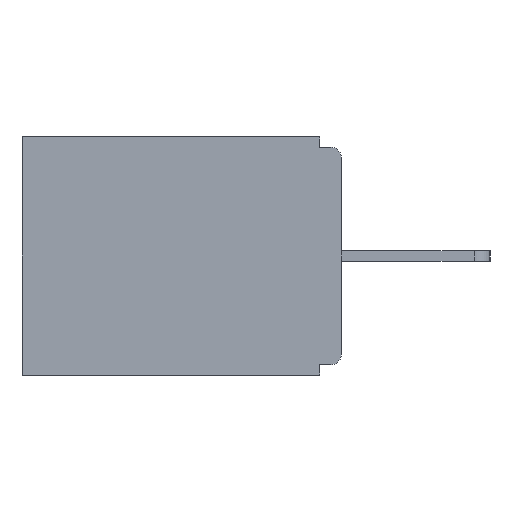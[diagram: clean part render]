
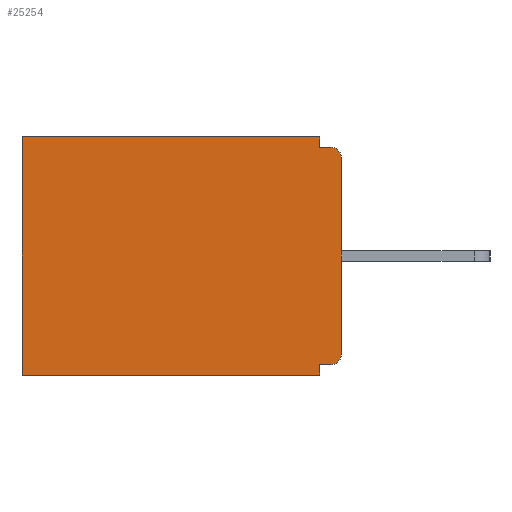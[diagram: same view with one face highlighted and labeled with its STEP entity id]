
A CAD part, left-side view. The second image highlights one B-rep face of the part: STEP entity #25254.
In plain terms, the highlighted planar face has unit normal (-1, 0, 0).
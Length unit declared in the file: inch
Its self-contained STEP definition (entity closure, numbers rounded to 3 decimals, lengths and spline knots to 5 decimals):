
#625 = DIRECTION ( 'NONE',  ( 0., 1., 0. ) ) ;
#708 = EDGE_CURVE ( 'NONE', #4098, #7398, #16030, .T. ) ;
#972 = PLANE ( 'NONE',  #22437 ) ;
#1460 = CARTESIAN_POINT ( 'NONE',  ( 0.298, 0., -0.343 ) ) ;
#1604 = VECTOR ( 'NONE', #17509, 39.37008 ) ;
#1806 = VECTOR ( 'NONE', #6865, 39.37008 ) ;
#1820 = DIRECTION ( 'NONE',  ( 0., 1., 0. ) ) ;
#1866 = ORIENTED_EDGE ( 'NONE', *, *, #15535, .F. ) ;
#1882 = EDGE_CURVE ( 'NONE', #14645, #4284, #15303, .T. ) ;
#1929 = CARTESIAN_POINT ( 'NONE',  ( 0.298, 0.015, -0.313 ) ) ;
#2220 = CARTESIAN_POINT ( 'NONE',  ( 0.298, 0.031, -0.015 ) ) ;
#2470 = EDGE_CURVE ( 'NONE', #3941, #7398, #4201, .T. ) ;
#2861 = DIRECTION ( 'NONE',  ( 0., 0., -1. ) ) ;
#2925 = DIRECTION ( 'NONE',  ( 0., 0., -1. ) ) ;
#3166 = FACE_OUTER_BOUND ( 'NONE', #17332, .T. ) ;
#3941 = VERTEX_POINT ( 'NONE', #17111 ) ;
#4076 = DIRECTION ( 'NONE',  ( 0., 0., -1. ) ) ;
#4098 = VERTEX_POINT ( 'NONE', #25697 ) ;
#4145 = ORIENTED_EDGE ( 'NONE', *, *, #6906, .T. ) ;
#4201 = LINE ( 'NONE', #1460, #8117 ) ;
#4284 = VERTEX_POINT ( 'NONE', #16744 ) ;
#4584 = VECTOR ( 'NONE', #2861, 39.37008 ) ;
#4990 = CARTESIAN_POINT ( 'NONE',  ( 0.298, 0.031, -0.328 ) ) ;
#4994 = ORIENTED_EDGE ( 'NONE', *, *, #20218, .F. ) ;
#5400 = CARTESIAN_POINT ( 'NONE',  ( 0.298, 0.46, -0.343 ) ) ;
#5636 = AXIS2_PLACEMENT_3D ( 'NONE', #26650, #8255, #4076 ) ;
#5731 = ORIENTED_EDGE ( 'NONE', *, *, #1882, .T. ) ;
#6865 = DIRECTION ( 'NONE',  ( 0., 0., -1. ) ) ;
#6906 = EDGE_CURVE ( 'NONE', #20373, #4098, #23483, .T. ) ;
#7398 = VERTEX_POINT ( 'NONE', #5400 ) ;
#8070 = ORIENTED_EDGE ( 'NONE', *, *, #24439, .F. ) ;
#8078 = ORIENTED_EDGE ( 'NONE', *, *, #12468, .F. ) ;
#8117 = VECTOR ( 'NONE', #1820, 39.37008 ) ;
#8255 = DIRECTION ( 'NONE',  ( -1., 0., 0. ) ) ;
#9333 = CARTESIAN_POINT ( 'NONE',  ( 0.298, 0., 0. ) ) ;
#10037 = CARTESIAN_POINT ( 'NONE',  ( 0.298, 0., -0.03 ) ) ;
#10203 = ORIENTED_EDGE ( 'NONE', *, *, #2470, .F. ) ;
#11081 = CARTESIAN_POINT ( 'NONE',  ( 0.298, 0.015, -0.015 ) ) ;
#11127 = VECTOR ( 'NONE', #625, 39.37008 ) ;
#11611 = DIRECTION ( 'NONE',  ( 0., -1., 0. ) ) ;
#11946 = VERTEX_POINT ( 'NONE', #10037 ) ;
#12468 = EDGE_CURVE ( 'NONE', #21699, #15199, #17417, .T. ) ;
#13054 = ORIENTED_EDGE ( 'NONE', *, *, #23594, .T. ) ;
#13057 = CARTESIAN_POINT ( 'NONE',  ( 0.298, 0., -0.328 ) ) ;
#13523 = CARTESIAN_POINT ( 'NONE',  ( 0.298, 0.031, -0.343 ) ) ;
#14033 = LINE ( 'NONE', #15560, #4584 ) ;
#14142 = CARTESIAN_POINT ( 'NONE',  ( 0.298, 0.015, -0.328 ) ) ;
#14493 = VECTOR ( 'NONE', #15778, 39.37008 ) ;
#14543 = CIRCLE ( 'NONE', #5636, 0.015 ) ;
#14645 = VERTEX_POINT ( 'NONE', #14142 ) ;
#15199 = VERTEX_POINT ( 'NONE', #11081 ) ;
#15303 = CIRCLE ( 'NONE', #17388, 0.015 ) ;
#15433 = CARTESIAN_POINT ( 'NONE',  ( 0.298, 0., 0. ) ) ;
#15535 = EDGE_CURVE ( 'NONE', #11946, #4284, #20571, .T. ) ;
#15560 = CARTESIAN_POINT ( 'NONE',  ( 0.298, 0.031, -0.343 ) ) ;
#15647 = CARTESIAN_POINT ( 'NONE',  ( 0.298, 0.031, 0. ) ) ;
#15778 = DIRECTION ( 'NONE',  ( 0., 1., 0. ) ) ;
#16030 = LINE ( 'NONE', #19454, #20532 ) ;
#16648 = LINE ( 'NONE', #13057, #11127 ) ;
#16744 = CARTESIAN_POINT ( 'NONE',  ( 0.298, 0., -0.313 ) ) ;
#17111 = CARTESIAN_POINT ( 'NONE',  ( 0.298, 0.031, -0.343 ) ) ;
#17332 = EDGE_LOOP ( 'NONE', ( #13054, #8078, #22883, #4145, #18236, #10203, #8070, #4994, #5731, #1866 ) ) ;
#17388 = AXIS2_PLACEMENT_3D ( 'NONE', #1929, #20527, #24654 ) ;
#17417 = LINE ( 'NONE', #23983, #24219 ) ;
#17509 = DIRECTION ( 'NONE',  ( 0., 0., -1. ) ) ;
#17537 = DIRECTION ( 'NONE',  ( 1., 0., 0. ) ) ;
#17762 = CARTESIAN_POINT ( 'NONE',  ( 0.298, 0., 0. ) ) ;
#18236 = ORIENTED_EDGE ( 'NONE', *, *, #708, .T. ) ;
#19454 = CARTESIAN_POINT ( 'NONE',  ( 0.298, 0.46, 0. ) ) ;
#19644 = DIRECTION ( 'NONE',  ( 0., 0., -1. ) ) ;
#20218 = EDGE_CURVE ( 'NONE', #14645, #25253, #16648, .T. ) ;
#20373 = VERTEX_POINT ( 'NONE', #15647 ) ;
#20424 = EDGE_CURVE ( 'NONE', #20373, #21699, #14033, .T. ) ;
#20527 = DIRECTION ( 'NONE',  ( -1., 0., 0. ) ) ;
#20532 = VECTOR ( 'NONE', #2925, 39.37008 ) ;
#20571 = LINE ( 'NONE', #9333, #1806 ) ;
#21671 = LINE ( 'NONE', #13523, #1604 ) ;
#21699 = VERTEX_POINT ( 'NONE', #2220 ) ;
#22437 = AXIS2_PLACEMENT_3D ( 'NONE', #15433, #17537, #19644 ) ;
#22883 = ORIENTED_EDGE ( 'NONE', *, *, #20424, .F. ) ;
#23483 = LINE ( 'NONE', #17762, #14493 ) ;
#23594 = EDGE_CURVE ( 'NONE', #11946, #15199, #14543, .T. ) ;
#23983 = CARTESIAN_POINT ( 'NONE',  ( 0.298, 0., -0.015 ) ) ;
#24219 = VECTOR ( 'NONE', #11611, 39.37008 ) ;
#24439 = EDGE_CURVE ( 'NONE', #25253, #3941, #21671, .T. ) ;
#24654 = DIRECTION ( 'NONE',  ( 0., 0., -1. ) ) ;
#25253 = VERTEX_POINT ( 'NONE', #4990 ) ;
#25254 = ADVANCED_FACE ( 'NONE', ( #3166 ), #972, .F. ) ;
#25697 = CARTESIAN_POINT ( 'NONE',  ( 0.298, 0.46, 0. ) ) ;
#26650 = CARTESIAN_POINT ( 'NONE',  ( 0.298, 0.015, -0.03 ) ) ;
